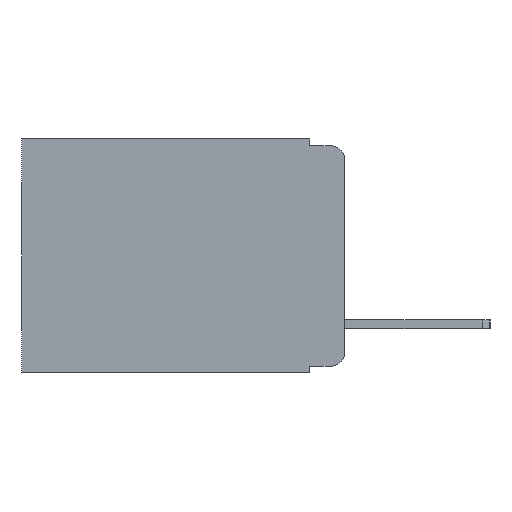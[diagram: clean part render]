
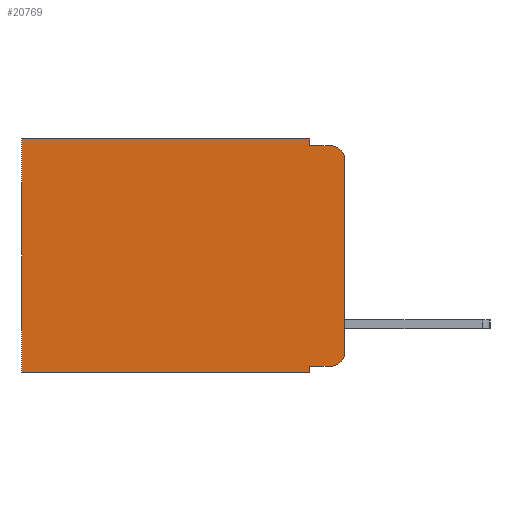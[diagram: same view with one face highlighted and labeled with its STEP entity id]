
A CAD part, left-side view. The second image highlights one B-rep face of the part: STEP entity #20769.
In plain terms, the highlighted planar face has unit normal (-1, 0, 0).
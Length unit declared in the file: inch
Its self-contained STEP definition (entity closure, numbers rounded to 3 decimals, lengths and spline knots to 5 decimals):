
#470 = CARTESIAN_POINT ( 'NONE',  ( 0.298, 0.051, -0.333 ) ) ;
#495 = LINE ( 'NONE', #17758, #20731 ) ;
#610 = ORIENTED_EDGE ( 'NONE', *, *, #16354, .F. ) ;
#987 = ORIENTED_EDGE ( 'NONE', *, *, #1054, .T. ) ;
#1054 = EDGE_CURVE ( 'NONE', #17761, #18040, #14592, .T. ) ;
#1157 = ORIENTED_EDGE ( 'NONE', *, *, #6614, .F. ) ;
#1328 = CIRCLE ( 'NONE', #7000, 0.02 ) ;
#1334 = VERTEX_POINT ( 'NONE', #18077 ) ;
#1454 = CARTESIAN_POINT ( 'NONE',  ( 0.298, 0.473, 0. ) ) ;
#1814 = VECTOR ( 'NONE', #9773, 39.37008 ) ;
#2111 = DIRECTION ( 'NONE',  ( 0., 0., -1. ) ) ;
#2181 = ORIENTED_EDGE ( 'NONE', *, *, #9723, .T. ) ;
#2348 = CARTESIAN_POINT ( 'NONE',  ( 0.298, 0., 0. ) ) ;
#2604 = CARTESIAN_POINT ( 'NONE',  ( 0.298, 0.051, -0.01 ) ) ;
#2634 = ORIENTED_EDGE ( 'NONE', *, *, #11131, .T. ) ;
#2857 = CARTESIAN_POINT ( 'NONE',  ( 0.298, 0.051, 0. ) ) ;
#3412 = CARTESIAN_POINT ( 'NONE',  ( 0.298, 0.051, -0.343 ) ) ;
#3538 = VECTOR ( 'NONE', #20251, 39.37008 ) ;
#3560 = VERTEX_POINT ( 'NONE', #3412 ) ;
#3993 = LINE ( 'NONE', #11164, #19854 ) ;
#4051 = VERTEX_POINT ( 'NONE', #6865 ) ;
#4198 = VERTEX_POINT ( 'NONE', #13217 ) ;
#4672 = VERTEX_POINT ( 'NONE', #2857 ) ;
#4960 = DIRECTION ( 'NONE',  ( 0., 1., 0. ) ) ;
#5014 = FACE_OUTER_BOUND ( 'NONE', #7428, .T. ) ;
#5094 = ORIENTED_EDGE ( 'NONE', *, *, #16088, .T. ) ;
#5311 = CARTESIAN_POINT ( 'NONE',  ( 0.298, 0., 0. ) ) ;
#5461 = CARTESIAN_POINT ( 'NONE',  ( 0.298, 0., -0.03 ) ) ;
#5505 = VECTOR ( 'NONE', #4960, 39.37008 ) ;
#5867 = EDGE_CURVE ( 'NONE', #4672, #16329, #20381, .T. ) ;
#6079 = VECTOR ( 'NONE', #19807, 39.37008 ) ;
#6116 = CARTESIAN_POINT ( 'NONE',  ( 0.298, 0.02, -0.03 ) ) ;
#6277 = CIRCLE ( 'NONE', #12648, 0.02 ) ;
#6399 = CARTESIAN_POINT ( 'NONE',  ( 0.298, 0.051, 0. ) ) ;
#6614 = EDGE_CURVE ( 'NONE', #17761, #3560, #3993, .T. ) ;
#6625 = DIRECTION ( 'NONE',  ( -1., 0., 0. ) ) ;
#6865 = CARTESIAN_POINT ( 'NONE',  ( 0.298, 0., -0.313 ) ) ;
#6968 = VERTEX_POINT ( 'NONE', #5461 ) ;
#7000 = AXIS2_PLACEMENT_3D ( 'NONE', #6116, #17115, #7725 ) ;
#7428 = EDGE_LOOP ( 'NONE', ( #8669, #5094, #12114, #15564, #19002, #2181, #610, #1157, #987, #2634 ) ) ;
#7725 = DIRECTION ( 'NONE',  ( 0., 0., -1. ) ) ;
#8669 = ORIENTED_EDGE ( 'NONE', *, *, #19254, .F. ) ;
#9642 = CARTESIAN_POINT ( 'NONE',  ( 0.298, 0., -0.343 ) ) ;
#9723 = EDGE_CURVE ( 'NONE', #16329, #14094, #495, .T. ) ;
#9773 = DIRECTION ( 'NONE',  ( 0., -1., 0. ) ) ;
#10018 = DIRECTION ( 'NONE',  ( 0., 0., -1. ) ) ;
#11131 = EDGE_CURVE ( 'NONE', #18040, #4051, #6277, .T. ) ;
#11164 = CARTESIAN_POINT ( 'NONE',  ( 0.298, 0.051, 0. ) ) ;
#11443 = PLANE ( 'NONE',  #12393 ) ;
#11803 = EDGE_CURVE ( 'NONE', #4672, #1334, #20493, .T. ) ;
#12114 = ORIENTED_EDGE ( 'NONE', *, *, #12858, .F. ) ;
#12393 = AXIS2_PLACEMENT_3D ( 'NONE', #5311, #19495, #10018 ) ;
#12454 = CARTESIAN_POINT ( 'NONE',  ( 0.298, 0., 0. ) ) ;
#12648 = AXIS2_PLACEMENT_3D ( 'NONE', #16030, #6625, #17625 ) ;
#12858 = EDGE_CURVE ( 'NONE', #1334, #4198, #17022, .T. ) ;
#13217 = CARTESIAN_POINT ( 'NONE',  ( 0.298, 0.02, -0.01 ) ) ;
#14094 = VERTEX_POINT ( 'NONE', #16783 ) ;
#14436 = LINE ( 'NONE', #2348, #6079 ) ;
#14592 = LINE ( 'NONE', #19558, #1814 ) ;
#15372 = DIRECTION ( 'NONE',  ( 0., -1., 0. ) ) ;
#15564 = ORIENTED_EDGE ( 'NONE', *, *, #11803, .F. ) ;
#15841 = VECTOR ( 'NONE', #18983, 39.37008 ) ;
#16030 = CARTESIAN_POINT ( 'NONE',  ( 0.298, 0.02, -0.313 ) ) ;
#16088 = EDGE_CURVE ( 'NONE', #6968, #4198, #1328, .T. ) ;
#16329 = VERTEX_POINT ( 'NONE', #1454 ) ;
#16354 = EDGE_CURVE ( 'NONE', #3560, #14094, #18580, .T. ) ;
#16531 = VECTOR ( 'NONE', #15372, 39.37008 ) ;
#16783 = CARTESIAN_POINT ( 'NONE',  ( 0.298, 0.473, -0.343 ) ) ;
#17022 = LINE ( 'NONE', #2604, #16531 ) ;
#17115 = DIRECTION ( 'NONE',  ( -1., 0., 0. ) ) ;
#17227 = CARTESIAN_POINT ( 'NONE',  ( 0.298, 0.02, -0.333 ) ) ;
#17625 = DIRECTION ( 'NONE',  ( 0., 0., -1. ) ) ;
#17758 = CARTESIAN_POINT ( 'NONE',  ( 0.298, 0.473, 0. ) ) ;
#17761 = VERTEX_POINT ( 'NONE', #470 ) ;
#18040 = VERTEX_POINT ( 'NONE', #17227 ) ;
#18077 = CARTESIAN_POINT ( 'NONE',  ( 0.298, 0.051, -0.01 ) ) ;
#18580 = LINE ( 'NONE', #9642, #5505 ) ;
#18983 = DIRECTION ( 'NONE',  ( 0., 0., -1. ) ) ;
#19002 = ORIENTED_EDGE ( 'NONE', *, *, #5867, .T. ) ;
#19254 = EDGE_CURVE ( 'NONE', #6968, #4051, #14436, .T. ) ;
#19332 = DIRECTION ( 'NONE',  ( 0., 0., -1. ) ) ;
#19495 = DIRECTION ( 'NONE',  ( 1., 0., 0. ) ) ;
#19558 = CARTESIAN_POINT ( 'NONE',  ( 0.298, 0.051, -0.333 ) ) ;
#19807 = DIRECTION ( 'NONE',  ( 0., 0., -1. ) ) ;
#19854 = VECTOR ( 'NONE', #2111, 39.37008 ) ;
#20251 = DIRECTION ( 'NONE',  ( 0., 1., 0. ) ) ;
#20381 = LINE ( 'NONE', #12454, #3538 ) ;
#20493 = LINE ( 'NONE', #6399, #15841 ) ;
#20731 = VECTOR ( 'NONE', #19332, 39.37008 ) ;
#20769 = ADVANCED_FACE ( 'NONE', ( #5014 ), #11443, .F. ) ;
